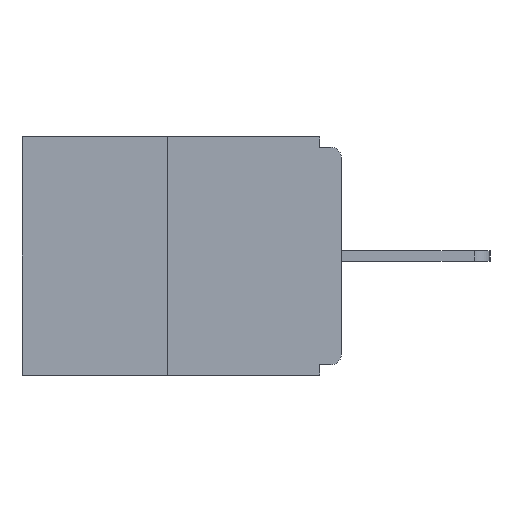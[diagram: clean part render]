
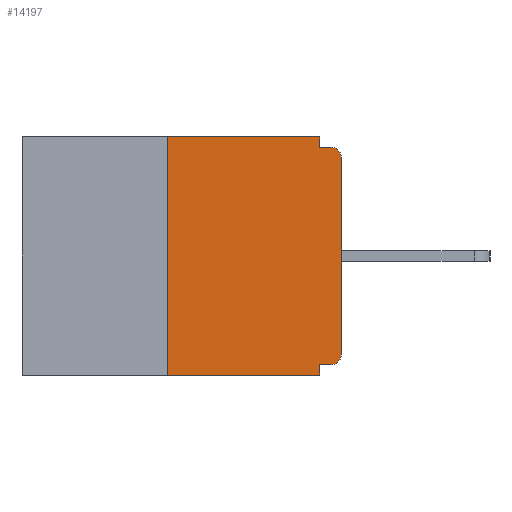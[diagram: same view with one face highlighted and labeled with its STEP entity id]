
A CAD part, left-side view. The second image highlights one B-rep face of the part: STEP entity #14197.
In plain terms, the highlighted planar face has unit normal (-1, 0, 0).
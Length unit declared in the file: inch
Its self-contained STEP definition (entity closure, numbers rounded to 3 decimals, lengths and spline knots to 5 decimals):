
#71 = ORIENTED_EDGE ( 'NONE', *, *, #1746, .T. ) ;
#381 = CARTESIAN_POINT ( 'NONE',  ( 0., 0., -0.015 ) ) ;
#457 = DIRECTION ( 'NONE',  ( 0., -1., 0. ) ) ;
#503 = CARTESIAN_POINT ( 'NONE',  ( 0., 0., -0.03 ) ) ;
#1150 = CARTESIAN_POINT ( 'NONE',  ( 0., 0.46, -0.343 ) ) ;
#1368 = VECTOR ( 'NONE', #6671, 39.37008 ) ;
#1738 = LINE ( 'NONE', #11625, #14328 ) ;
#1746 = EDGE_CURVE ( 'NONE', #6924, #15333, #12598, .T. ) ;
#1811 = VECTOR ( 'NONE', #14782, 39.37008 ) ;
#1816 = PLANE ( 'NONE',  #6597 ) ;
#1882 = LINE ( 'NONE', #10286, #1368 ) ;
#2157 = VERTEX_POINT ( 'NONE', #4787 ) ;
#2612 = CARTESIAN_POINT ( 'NONE',  ( 0., 0.031, -0.015 ) ) ;
#2683 = CIRCLE ( 'NONE', #5836, 0.015 ) ;
#2817 = FACE_OUTER_BOUND ( 'NONE', #3063, .T. ) ;
#3063 = EDGE_LOOP ( 'NONE', ( #14579, #10252, #3512, #5778, #11067, #14692, #11539, #71, #6064, #6294 ) ) ;
#3512 = ORIENTED_EDGE ( 'NONE', *, *, #5920, .T. ) ;
#3635 = LINE ( 'NONE', #1150, #12470 ) ;
#3662 = VECTOR ( 'NONE', #11222, 39.37008 ) ;
#4169 = CARTESIAN_POINT ( 'NONE',  ( 0., 0.25, -0.343 ) ) ;
#4361 = CARTESIAN_POINT ( 'NONE',  ( 0., 0.25, 0. ) ) ;
#4476 = CARTESIAN_POINT ( 'NONE',  ( 0., 0.015, -0.313 ) ) ;
#4732 = CARTESIAN_POINT ( 'NONE',  ( 0., 0.031, 0. ) ) ;
#4787 = CARTESIAN_POINT ( 'NONE',  ( 0., 0.031, -0.343 ) ) ;
#4882 = LINE ( 'NONE', #6365, #3662 ) ;
#5554 = EDGE_CURVE ( 'NONE', #12089, #14690, #1738, .T. ) ;
#5778 = ORIENTED_EDGE ( 'NONE', *, *, #16010, .F. ) ;
#5836 = AXIS2_PLACEMENT_3D ( 'NONE', #4476, #15583, #11811 ) ;
#5920 = EDGE_CURVE ( 'NONE', #9597, #2157, #3635, .T. ) ;
#6064 = ORIENTED_EDGE ( 'NONE', *, *, #8887, .F. ) ;
#6187 = DIRECTION ( 'NONE',  ( 0., -1., 0. ) ) ;
#6294 = ORIENTED_EDGE ( 'NONE', *, *, #11013, .F. ) ;
#6365 = CARTESIAN_POINT ( 'NONE',  ( 0., 0., -0.328 ) ) ;
#6511 = DIRECTION ( 'NONE',  ( 0., 0., 1. ) ) ;
#6597 = AXIS2_PLACEMENT_3D ( 'NONE', #14411, #6843, #15560 ) ;
#6671 = DIRECTION ( 'NONE',  ( 0., 0., -1. ) ) ;
#6843 = DIRECTION ( 'NONE',  ( 1., 0., 0. ) ) ;
#6924 = VERTEX_POINT ( 'NONE', #503 ) ;
#7058 = VERTEX_POINT ( 'NONE', #15954 ) ;
#7598 = AXIS2_PLACEMENT_3D ( 'NONE', #15450, #15214, #11677 ) ;
#7760 = DIRECTION ( 'NONE',  ( 0., -1., 0. ) ) ;
#7761 = VERTEX_POINT ( 'NONE', #2612 ) ;
#7916 = CARTESIAN_POINT ( 'NONE',  ( 0., 0.25, 0. ) ) ;
#8887 = EDGE_CURVE ( 'NONE', #7761, #15333, #9364, .T. ) ;
#9006 = EDGE_CURVE ( 'NONE', #12581, #6924, #9960, .T. ) ;
#9153 = LINE ( 'NONE', #7916, #13677 ) ;
#9364 = LINE ( 'NONE', #381, #16179 ) ;
#9597 = VERTEX_POINT ( 'NONE', #4169 ) ;
#9960 = LINE ( 'NONE', #12669, #10442 ) ;
#10252 = ORIENTED_EDGE ( 'NONE', *, *, #14183, .F. ) ;
#10286 = CARTESIAN_POINT ( 'NONE',  ( 0., 0.031, -0.343 ) ) ;
#10442 = VECTOR ( 'NONE', #6511, 39.37008 ) ;
#10742 = VERTEX_POINT ( 'NONE', #12438 ) ;
#11013 = EDGE_CURVE ( 'NONE', #14690, #7761, #15983, .T. ) ;
#11067 = ORIENTED_EDGE ( 'NONE', *, *, #11533, .F. ) ;
#11222 = DIRECTION ( 'NONE',  ( 0., 1., 0. ) ) ;
#11533 = EDGE_CURVE ( 'NONE', #7058, #10742, #4882, .T. ) ;
#11539 = ORIENTED_EDGE ( 'NONE', *, *, #9006, .T. ) ;
#11625 = CARTESIAN_POINT ( 'NONE',  ( 0., 0.46, 0. ) ) ;
#11677 = DIRECTION ( 'NONE',  ( 0., 0., -1. ) ) ;
#11757 = CARTESIAN_POINT ( 'NONE',  ( 0., 0., -0.313 ) ) ;
#11811 = DIRECTION ( 'NONE',  ( 0., 0., -1. ) ) ;
#12089 = VERTEX_POINT ( 'NONE', #4361 ) ;
#12438 = CARTESIAN_POINT ( 'NONE',  ( 0., 0.031, -0.328 ) ) ;
#12470 = VECTOR ( 'NONE', #6187, 39.37008 ) ;
#12581 = VERTEX_POINT ( 'NONE', #11757 ) ;
#12598 = CIRCLE ( 'NONE', #7598, 0.015 ) ;
#12669 = CARTESIAN_POINT ( 'NONE',  ( 0., 0., 0. ) ) ;
#13677 = VECTOR ( 'NONE', #14094, 39.37008 ) ;
#14094 = DIRECTION ( 'NONE',  ( 0., 0., 1. ) ) ;
#14183 = EDGE_CURVE ( 'NONE', #9597, #12089, #9153, .T. ) ;
#14197 = ADVANCED_FACE ( 'NONE', ( #2817 ), #1816, .F. ) ;
#14328 = VECTOR ( 'NONE', #7760, 39.37008 ) ;
#14411 = CARTESIAN_POINT ( 'NONE',  ( 0., 0.46, 0. ) ) ;
#14579 = ORIENTED_EDGE ( 'NONE', *, *, #5554, .F. ) ;
#14636 = CARTESIAN_POINT ( 'NONE',  ( 0., 0.031, 0. ) ) ;
#14690 = VERTEX_POINT ( 'NONE', #14636 ) ;
#14692 = ORIENTED_EDGE ( 'NONE', *, *, #15591, .T. ) ;
#14782 = DIRECTION ( 'NONE',  ( 0., 0., -1. ) ) ;
#14858 = CARTESIAN_POINT ( 'NONE',  ( 0., 0.015, -0.015 ) ) ;
#15214 = DIRECTION ( 'NONE',  ( -1., 0., 0. ) ) ;
#15333 = VERTEX_POINT ( 'NONE', #14858 ) ;
#15450 = CARTESIAN_POINT ( 'NONE',  ( 0., 0.015, -0.03 ) ) ;
#15560 = DIRECTION ( 'NONE',  ( 0., 0., -1. ) ) ;
#15583 = DIRECTION ( 'NONE',  ( -1., 0., 0. ) ) ;
#15591 = EDGE_CURVE ( 'NONE', #7058, #12581, #2683, .T. ) ;
#15954 = CARTESIAN_POINT ( 'NONE',  ( 0., 0.015, -0.328 ) ) ;
#15983 = LINE ( 'NONE', #4732, #1811 ) ;
#16010 = EDGE_CURVE ( 'NONE', #10742, #2157, #1882, .T. ) ;
#16179 = VECTOR ( 'NONE', #457, 39.37008 ) ;
